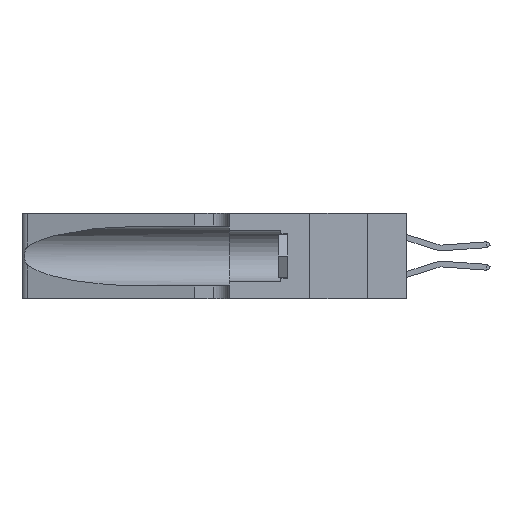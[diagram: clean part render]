
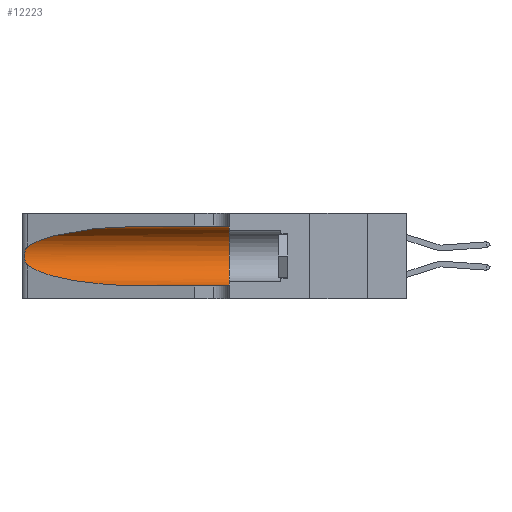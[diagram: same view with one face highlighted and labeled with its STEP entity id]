
A CAD part, left-side view. The second image highlights one B-rep face of the part: STEP entity #12223.
In plain terms, the highlighted cylindrical face has radius 3.308 mm (diameter 6.617 mm), a partial arc.
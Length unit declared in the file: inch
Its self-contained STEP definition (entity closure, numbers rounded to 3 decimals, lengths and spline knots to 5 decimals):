
#72 = DIRECTION ( 'NONE',  ( 0., -1., 0. ) ) ;
#89 = EDGE_CURVE ( 'NONE', #24010, #16212, #11044, .T. ) ;
#644 = DIRECTION ( 'NONE',  ( 0., -1., 0. ) ) ;
#1002 = CARTESIAN_POINT ( 'NONE',  ( 0.1305, 1.61858, 0.31525 ) ) ;
#1342 = CARTESIAN_POINT ( 'NONE',  ( 0.25487, 1.22718, 0.14631 ) ) ;
#1549 = EDGE_CURVE ( 'NONE', #11338, #1594, #8804, .T. ) ;
#1594 = VERTEX_POINT ( 'NONE', #7861 ) ;
#3528 = CARTESIAN_POINT ( 'NONE',  ( 0.1305, 0.35, 0.05475 ) ) ;
#4157 = DIRECTION ( 'NONE',  ( 0., 0., 1. ) ) ;
#4219 = CARTESIAN_POINT ( 'NONE',  ( 0.2373, 1.15595, 0.08982 ) ) ;
#5278 = ORIENTED_EDGE ( 'NONE', *, *, #18519, .T. ) ;
#5550 = CARTESIAN_POINT ( 'NONE',  ( 0.25487, 1.22718, 0.22369 ) ) ;
#5924 = VERTEX_POINT ( 'NONE', #13190 ) ;
#6148 = CARTESIAN_POINT ( 'NONE',  ( 0.25487, 1.22718, 0.14631 ) ) ;
#6225 = CARTESIAN_POINT ( 'NONE',  ( 0.1305, 1.61858, 0.05475 ) ) ;
#6628 = CARTESIAN_POINT ( 'NONE',  ( 0.1305, 0.35, 0.31525 ) ) ;
#7321 = CARTESIAN_POINT ( 'NONE',  ( 0.25789, 1.23486, 0.15765 ) ) ;
#7699 = ORIENTED_EDGE ( 'NONE', *, *, #23974, .F. ) ;
#7725 = CARTESIAN_POINT ( 'NONE',  ( 0.1305, 0.35, 0.185 ) ) ;
#7861 = CARTESIAN_POINT ( 'NONE',  ( 0.1305, 0.72297, 0.05475 ) ) ;
#7919 = ORIENTED_EDGE ( 'NONE', *, *, #1549, .T. ) ;
#8804 =( BOUNDED_CURVE ( )  B_SPLINE_CURVE ( 3, ( #18186, #4219, #12044, #21985 ),
 .UNSPECIFIED., .F., .F. ) 
 B_SPLINE_CURVE_WITH_KNOTS ( ( 4, 4 ),
 ( 3.44316, 4.71239 ),
 .UNSPECIFIED. ) 
 CURVE ( )  GEOMETRIC_REPRESENTATION_ITEM ( )  RATIONAL_B_SPLINE_CURVE ( ( 1., 0.87, 0.87, 1. ) ) 
 REPRESENTATION_ITEM ( '' )  );
#9465 = CARTESIAN_POINT ( 'NONE',  ( 0.25555, 1.22994, 0.2215 ) ) ;
#9535 = CARTESIAN_POINT ( 'NONE',  ( 0.26075, 1.23896, 0.19203 ) ) ;
#10373 = CARTESIAN_POINT ( 'NONE',  ( 0.1305, 1.61858, 0.185 ) ) ;
#11044 = CIRCLE ( 'NONE', #23789, 0.13025 ) ;
#11166 = CARTESIAN_POINT ( 'NONE',  ( 0.25555, 1.22993, 0.14849 ) ) ;
#11338 = VERTEX_POINT ( 'NONE', #6148 ) ;
#11609 = VERTEX_POINT ( 'NONE', #24933 ) ;
#12044 = CARTESIAN_POINT ( 'NONE',  ( 0.18966, 0.96281, 0.05475 ) ) ;
#12223 = ADVANCED_FACE ( 'NONE', ( #20312 ), #17842, .F. ) ;
#12340 = DIRECTION ( 'NONE',  ( 0., 0., -1. ) ) ;
#13144 = CARTESIAN_POINT ( 'NONE',  ( 0.25639, 1.23186, 0.15144 ) ) ;
#13190 = CARTESIAN_POINT ( 'NONE',  ( 0.25487, 1.22718, 0.22369 ) ) ;
#13219 = DIRECTION ( 'NONE',  ( 0., 1., 0. ) ) ;
#14065 = ORIENTED_EDGE ( 'NONE', *, *, #20096, .T. ) ;
#14764 =( BOUNDED_CURVE ( )  B_SPLINE_CURVE ( 3, ( #15184, #17160, #21157, #25148 ),
 .UNSPECIFIED., .F., .F. ) 
 B_SPLINE_CURVE_WITH_KNOTS ( ( 4, 4 ),
 ( 1.5708, 2.84003 ),
 .UNSPECIFIED. ) 
 CURVE ( )  GEOMETRIC_REPRESENTATION_ITEM ( )  RATIONAL_B_SPLINE_CURVE ( ( 1., 0.87, 0.87, 1. ) ) 
 REPRESENTATION_ITEM ( '' )  );
#14931 = VECTOR ( 'NONE', #644, 39.37008 ) ;
#15170 = AXIS2_PLACEMENT_3D ( 'NONE', #10373, #24219, #12340 ) ;
#15184 = CARTESIAN_POINT ( 'NONE',  ( 0.1305, 0.72297, 0.31525 ) ) ;
#16212 = VERTEX_POINT ( 'NONE', #3528 ) ;
#17025 = CARTESIAN_POINT ( 'NONE',  ( 0.25639, 1.23184, 0.21858 ) ) ;
#17160 = CARTESIAN_POINT ( 'NONE',  ( 0.18966, 0.96281, 0.31525 ) ) ;
#17842 = CYLINDRICAL_SURFACE ( 'NONE', #15170, 0.13025 ) ;
#18186 = CARTESIAN_POINT ( 'NONE',  ( 0.25487, 1.22718, 0.14631 ) ) ;
#18519 = EDGE_CURVE ( 'NONE', #1594, #16212, #20482, .T. ) ;
#19134 = ORIENTED_EDGE ( 'NONE', *, *, #89, .F. ) ;
#19358 = CARTESIAN_POINT ( 'NONE',  ( 0.26018, 1.23835, 0.19895 ) ) ;
#19578 = LINE ( 'NONE', #1002, #14931 ) ;
#20096 = EDGE_CURVE ( 'NONE', #5924, #11338, #22381, .T. ) ;
#20312 = FACE_OUTER_BOUND ( 'NONE', #25489, .T. ) ;
#20482 = LINE ( 'NONE', #6225, #21749 ) ;
#21157 = CARTESIAN_POINT ( 'NONE',  ( 0.2373, 1.15595, 0.28018 ) ) ;
#21527 = EDGE_CURVE ( 'NONE', #11609, #5924, #14764, .T. ) ;
#21749 = VECTOR ( 'NONE', #72, 39.37008 ) ;
#21985 = CARTESIAN_POINT ( 'NONE',  ( 0.1305, 0.72297, 0.05475 ) ) ;
#22381 = B_SPLINE_CURVE_WITH_KNOTS ( 'NONE', 3,
 ( #5550, #9465, #17025, #23104, #23281, #19358, #9535, #23367, #24931, #23013, #7321, #13144, #11166, #1342 ),
 .UNSPECIFIED., .F., .F.,
 ( 4, 2, 2, 2, 2, 2, 4 ),
 ( 0., 0.00027, 0.00053, 0.00107, 0.0016, 0.00187, 0.00214 ),
 .UNSPECIFIED. ) ;
#23013 = CARTESIAN_POINT ( 'NONE',  ( 0.25856, 1.23593, 0.16098 ) ) ;
#23104 = CARTESIAN_POINT ( 'NONE',  ( 0.25787, 1.23484, 0.2124 ) ) ;
#23281 = CARTESIAN_POINT ( 'NONE',  ( 0.25854, 1.2359, 0.20912 ) ) ;
#23367 = CARTESIAN_POINT ( 'NONE',  ( 0.26075, 1.23896, 0.178 ) ) ;
#23789 = AXIS2_PLACEMENT_3D ( 'NONE', #7725, #13219, #4157 ) ;
#23974 = EDGE_CURVE ( 'NONE', #11609, #24010, #19578, .T. ) ;
#24010 = VERTEX_POINT ( 'NONE', #6628 ) ;
#24219 = DIRECTION ( 'NONE',  ( 0., -1., 0. ) ) ;
#24414 = ORIENTED_EDGE ( 'NONE', *, *, #21527, .T. ) ;
#24931 = CARTESIAN_POINT ( 'NONE',  ( 0.26017, 1.23833, 0.17102 ) ) ;
#24933 = CARTESIAN_POINT ( 'NONE',  ( 0.1305, 0.72297, 0.31525 ) ) ;
#25148 = CARTESIAN_POINT ( 'NONE',  ( 0.25487, 1.22718, 0.22369 ) ) ;
#25489 = EDGE_LOOP ( 'NONE', ( #24414, #14065, #7919, #5278, #19134, #7699 ) ) ;
